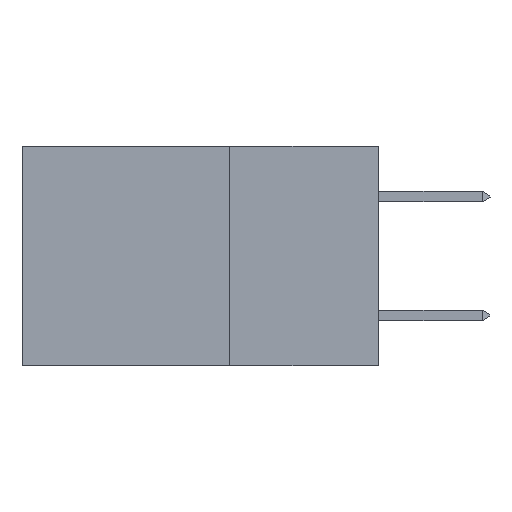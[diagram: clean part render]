
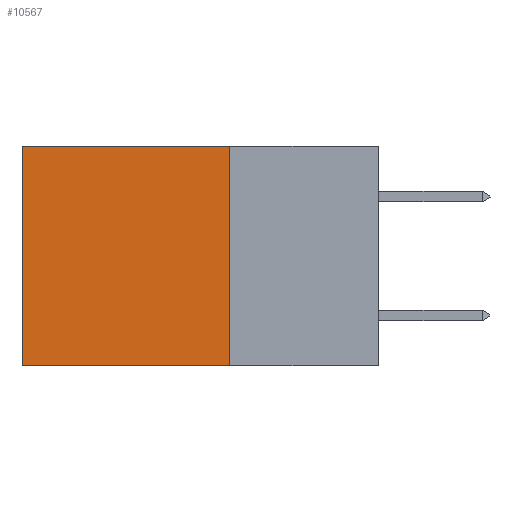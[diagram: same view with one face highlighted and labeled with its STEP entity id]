
A CAD part, left-side view. The second image highlights one B-rep face of the part: STEP entity #10567.
In plain terms, the highlighted planar face has unit normal (-1, 0, 0).
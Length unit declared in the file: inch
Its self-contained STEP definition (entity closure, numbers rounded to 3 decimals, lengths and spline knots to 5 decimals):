
#677 = EDGE_CURVE ( 'NONE', #17230, #18458, #2670, .T. ) ;
#678 = VECTOR ( 'NONE', #24087, 39.37008 ) ;
#2431 = PLANE ( 'NONE',  #11060 ) ;
#2670 = LINE ( 'NONE', #7883, #23636 ) ;
#3393 = VECTOR ( 'NONE', #24225, 39.37008 ) ;
#3478 = CARTESIAN_POINT ( 'NONE',  ( 0.298, 0.6, 0. ) ) ;
#4118 = VERTEX_POINT ( 'NONE', #7076 ) ;
#4895 = CARTESIAN_POINT ( 'NONE',  ( 0.298, 0.25, 0. ) ) ;
#5810 = ORIENTED_EDGE ( 'NONE', *, *, #18606, .F. ) ;
#6574 = ORIENTED_EDGE ( 'NONE', *, *, #19033, .T. ) ;
#7044 = ORIENTED_EDGE ( 'NONE', *, *, #677, .T. ) ;
#7076 = CARTESIAN_POINT ( 'NONE',  ( 0.298, 0.6, -0.37 ) ) ;
#7673 = EDGE_CURVE ( 'NONE', #17230, #18621, #19433, .T. ) ;
#7883 = CARTESIAN_POINT ( 'NONE',  ( 0.298, 0.25, 0. ) ) ;
#8211 = CARTESIAN_POINT ( 'NONE',  ( 0.298, 0.25, 0. ) ) ;
#9352 = FACE_OUTER_BOUND ( 'NONE', #18124, .T. ) ;
#9611 = ORIENTED_EDGE ( 'NONE', *, *, #7673, .F. ) ;
#10567 = ADVANCED_FACE ( 'NONE', ( #9352 ), #2431, .F. ) ;
#11060 = AXIS2_PLACEMENT_3D ( 'NONE', #4895, #18491, #20710 ) ;
#11134 = CARTESIAN_POINT ( 'NONE',  ( 0.298, 0.6, 0. ) ) ;
#11667 = LINE ( 'NONE', #11134, #22174 ) ;
#11998 = CARTESIAN_POINT ( 'NONE',  ( 0.298, 0.25, 0. ) ) ;
#14165 = LINE ( 'NONE', #22017, #3393 ) ;
#17230 = VERTEX_POINT ( 'NONE', #8211 ) ;
#18124 = EDGE_LOOP ( 'NONE', ( #6574, #5810, #9611, #7044 ) ) ;
#18458 = VERTEX_POINT ( 'NONE', #3478 ) ;
#18491 = DIRECTION ( 'NONE',  ( 1., 0., 0. ) ) ;
#18606 = EDGE_CURVE ( 'NONE', #18621, #4118, #14165, .T. ) ;
#18621 = VERTEX_POINT ( 'NONE', #19891 ) ;
#19033 = EDGE_CURVE ( 'NONE', #18458, #4118, #11667, .T. ) ;
#19433 = LINE ( 'NONE', #11998, #678 ) ;
#19683 = DIRECTION ( 'NONE',  ( 0., 0., -1. ) ) ;
#19891 = CARTESIAN_POINT ( 'NONE',  ( 0.298, 0.25, -0.37 ) ) ;
#20691 = DIRECTION ( 'NONE',  ( 0., 1., 0. ) ) ;
#20710 = DIRECTION ( 'NONE',  ( 0., 0., -1. ) ) ;
#22017 = CARTESIAN_POINT ( 'NONE',  ( 0.298, 0.25, -0.37 ) ) ;
#22174 = VECTOR ( 'NONE', #19683, 39.37008 ) ;
#23636 = VECTOR ( 'NONE', #20691, 39.37008 ) ;
#24087 = DIRECTION ( 'NONE',  ( 0., 0., -1. ) ) ;
#24225 = DIRECTION ( 'NONE',  ( 0., 1., 0. ) ) ;
